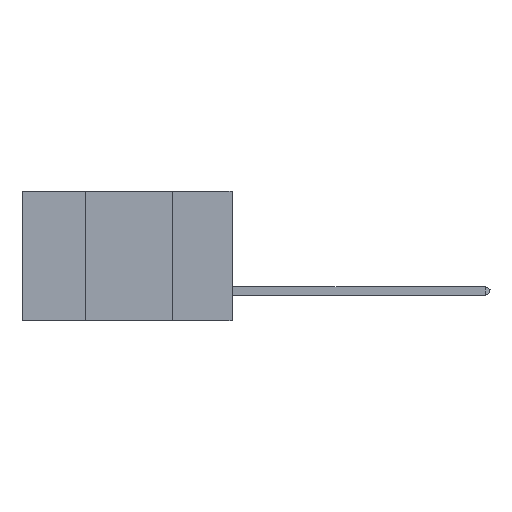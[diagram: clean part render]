
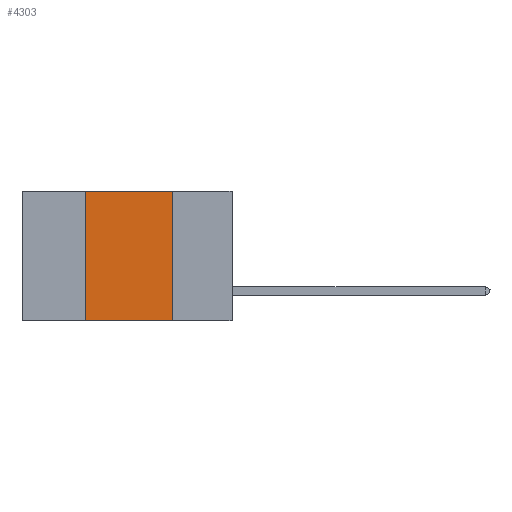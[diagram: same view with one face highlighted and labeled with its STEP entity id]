
A CAD part, left-side view. The second image highlights one B-rep face of the part: STEP entity #4303.
In plain terms, the highlighted planar face has unit normal (-1, 0, 0).
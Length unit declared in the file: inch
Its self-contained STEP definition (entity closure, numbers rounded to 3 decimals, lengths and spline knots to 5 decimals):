
#10 = CARTESIAN_POINT ( 'NONE',  ( 0., 0.42, -0.37 ) ) ;
#624 = CARTESIAN_POINT ( 'NONE',  ( 0., 0.6, 0. ) ) ;
#982 = VERTEX_POINT ( 'NONE', #10 ) ;
#1353 = ORIENTED_EDGE ( 'NONE', *, *, #11663, .T. ) ;
#2553 = LINE ( 'NONE', #12271, #14218 ) ;
#4303 = ADVANCED_FACE ( 'NONE', ( #18201 ), #4861, .F. ) ;
#4495 = EDGE_CURVE ( 'NONE', #982, #21093, #15761, .T. ) ;
#4861 = PLANE ( 'NONE',  #22283 ) ;
#5001 = VERTEX_POINT ( 'NONE', #11700 ) ;
#6154 = LINE ( 'NONE', #624, #21951 ) ;
#6459 = DIRECTION ( 'NONE',  ( 0., 0., -1. ) ) ;
#6712 = ORIENTED_EDGE ( 'NONE', *, *, #12947, .F. ) ;
#9223 = CARTESIAN_POINT ( 'NONE',  ( 0., 0.17, 0. ) ) ;
#9560 = DIRECTION ( 'NONE',  ( 0., -1., 0. ) ) ;
#10019 = VERTEX_POINT ( 'NONE', #9223 ) ;
#10345 = DIRECTION ( 'NONE',  ( 0., -1., 0. ) ) ;
#11663 = EDGE_CURVE ( 'NONE', #982, #5001, #2553, .T. ) ;
#11700 = CARTESIAN_POINT ( 'NONE',  ( 0., 0.17, -0.37 ) ) ;
#11958 = CARTESIAN_POINT ( 'NONE',  ( 0., 0.42, 0. ) ) ;
#11975 = DIRECTION ( 'NONE',  ( 0., 0., -1. ) ) ;
#12249 = LINE ( 'NONE', #22331, #19142 ) ;
#12271 = CARTESIAN_POINT ( 'NONE',  ( 0., 0.6, -0.37 ) ) ;
#12947 = EDGE_CURVE ( 'NONE', #10019, #5001, #12249, .T. ) ;
#13530 = DIRECTION ( 'NONE',  ( 1., 0., 0. ) ) ;
#13668 = DIRECTION ( 'NONE',  ( 0., 0., 1. ) ) ;
#14218 = VECTOR ( 'NONE', #10345, 39.37008 ) ;
#15680 = CARTESIAN_POINT ( 'NONE',  ( 0., 0.42, 0. ) ) ;
#15681 = ORIENTED_EDGE ( 'NONE', *, *, #20260, .F. ) ;
#15761 = LINE ( 'NONE', #15680, #18761 ) ;
#16063 = ORIENTED_EDGE ( 'NONE', *, *, #4495, .F. ) ;
#17581 = EDGE_LOOP ( 'NONE', ( #6712, #15681, #16063, #1353 ) ) ;
#18201 = FACE_OUTER_BOUND ( 'NONE', #17581, .T. ) ;
#18761 = VECTOR ( 'NONE', #13668, 39.37008 ) ;
#19142 = VECTOR ( 'NONE', #6459, 39.37008 ) ;
#20260 = EDGE_CURVE ( 'NONE', #21093, #10019, #6154, .T. ) ;
#21093 = VERTEX_POINT ( 'NONE', #11958 ) ;
#21951 = VECTOR ( 'NONE', #9560, 39.37008 ) ;
#22283 = AXIS2_PLACEMENT_3D ( 'NONE', #22464, #13530, #11975 ) ;
#22331 = CARTESIAN_POINT ( 'NONE',  ( 0., 0.17, 0. ) ) ;
#22464 = CARTESIAN_POINT ( 'NONE',  ( 0., 0.6, 0. ) ) ;
